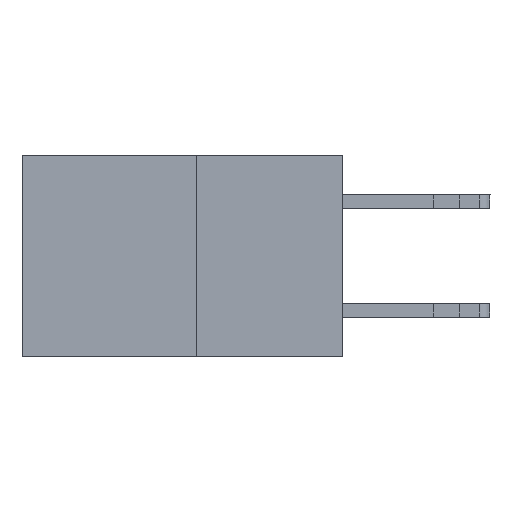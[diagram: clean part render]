
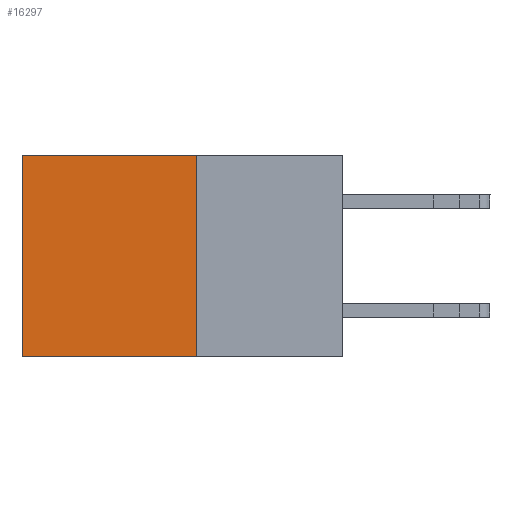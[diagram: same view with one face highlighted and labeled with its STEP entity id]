
A CAD part, left-side view. The second image highlights one B-rep face of the part: STEP entity #16297.
In plain terms, the highlighted planar face has unit normal (-1, 0, 0).
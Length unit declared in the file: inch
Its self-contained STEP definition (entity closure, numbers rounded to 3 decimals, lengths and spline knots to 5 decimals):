
#4 = ORIENTED_EDGE ( 'NONE', *, *, #9563, .T. ) ;
#666 = VERTEX_POINT ( 'NONE', #14573 ) ;
#776 = VERTEX_POINT ( 'NONE', #9864 ) ;
#1526 = FACE_OUTER_BOUND ( 'NONE', #17539, .T. ) ;
#1597 = AXIS2_PLACEMENT_3D ( 'NONE', #2829, #7751, #18954 ) ;
#1917 = CARTESIAN_POINT ( 'NONE',  ( 0.277, 0.59, -0.37 ) ) ;
#2200 = LINE ( 'NONE', #18842, #11313 ) ;
#2829 = CARTESIAN_POINT ( 'NONE',  ( 0.277, 0.27, -0.37 ) ) ;
#2885 = CARTESIAN_POINT ( 'NONE',  ( 0.277, 0.59, -0.37 ) ) ;
#2976 = CARTESIAN_POINT ( 'NONE',  ( 0.277, 0.27, -0.37 ) ) ;
#3537 = DIRECTION ( 'NONE',  ( 0., 0., -1. ) ) ;
#4306 = LINE ( 'NONE', #1917, #12339 ) ;
#4597 = DIRECTION ( 'NONE',  ( 0., 1., 0. ) ) ;
#7751 = DIRECTION ( 'NONE',  ( 1., 0., 0. ) ) ;
#7988 = DIRECTION ( 'NONE',  ( 0., 1., 0. ) ) ;
#8014 = CARTESIAN_POINT ( 'NONE',  ( 0.277, 0.27, 0. ) ) ;
#8631 = VECTOR ( 'NONE', #4597, 39.37008 ) ;
#9563 = EDGE_CURVE ( 'NONE', #776, #14095, #16618, .T. ) ;
#9864 = CARTESIAN_POINT ( 'NONE',  ( 0.277, 0.27, 0. ) ) ;
#11313 = VECTOR ( 'NONE', #12417, 39.37008 ) ;
#11386 = VECTOR ( 'NONE', #7988, 39.37008 ) ;
#11758 = EDGE_CURVE ( 'NONE', #776, #666, #2200, .T. ) ;
#12339 = VECTOR ( 'NONE', #3537, 39.37008 ) ;
#12417 = DIRECTION ( 'NONE',  ( 0., 0., -1. ) ) ;
#12464 = PLANE ( 'NONE',  #1597 ) ;
#14095 = VERTEX_POINT ( 'NONE', #16983 ) ;
#14573 = CARTESIAN_POINT ( 'NONE',  ( 0.277, 0.27, -0.37 ) ) ;
#15154 = EDGE_CURVE ( 'NONE', #14095, #19645, #4306, .T. ) ;
#16297 = ADVANCED_FACE ( 'NONE', ( #1526 ), #12464, .F. ) ;
#16335 = EDGE_CURVE ( 'NONE', #666, #19645, #17106, .T. ) ;
#16618 = LINE ( 'NONE', #8014, #11386 ) ;
#16983 = CARTESIAN_POINT ( 'NONE',  ( 0.277, 0.59, 0. ) ) ;
#17106 = LINE ( 'NONE', #2976, #8631 ) ;
#17539 = EDGE_LOOP ( 'NONE', ( #20058, #20286, #20512, #4 ) ) ;
#18842 = CARTESIAN_POINT ( 'NONE',  ( 0.277, 0.27, -0.37 ) ) ;
#18954 = DIRECTION ( 'NONE',  ( 0., 0., -1. ) ) ;
#19645 = VERTEX_POINT ( 'NONE', #2885 ) ;
#20058 = ORIENTED_EDGE ( 'NONE', *, *, #15154, .T. ) ;
#20286 = ORIENTED_EDGE ( 'NONE', *, *, #16335, .F. ) ;
#20512 = ORIENTED_EDGE ( 'NONE', *, *, #11758, .F. ) ;
